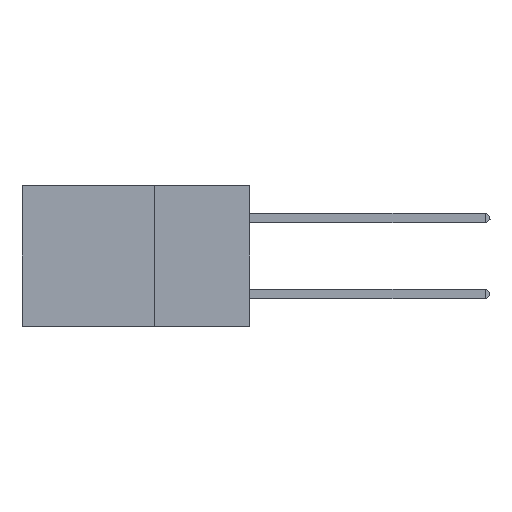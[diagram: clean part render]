
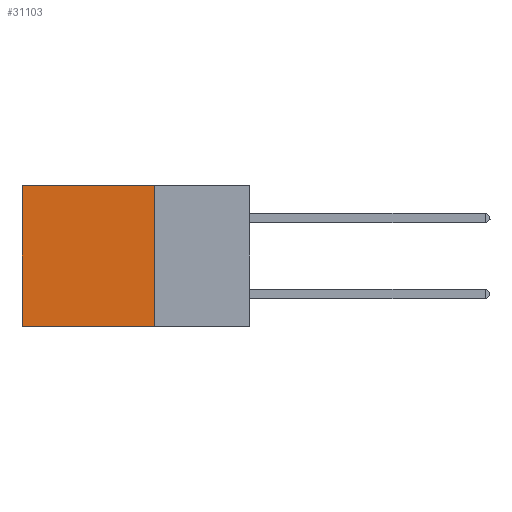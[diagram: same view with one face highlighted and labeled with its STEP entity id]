
A CAD part, left-side view. The second image highlights one B-rep face of the part: STEP entity #31103.
In plain terms, the highlighted planar face has unit normal (-1, 0, 0).
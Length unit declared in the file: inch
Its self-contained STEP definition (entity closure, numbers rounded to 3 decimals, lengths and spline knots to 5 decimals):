
#196 = DIRECTION ( 'NONE',  ( 0., 0., -1. ) ) ;
#592 = DIRECTION ( 'NONE',  ( 0., 0., -1. ) ) ;
#1498 = VERTEX_POINT ( 'NONE', #19120 ) ;
#3432 = EDGE_CURVE ( 'NONE', #1498, #26394, #28209, .T. ) ;
#7905 = AXIS2_PLACEMENT_3D ( 'NONE', #16651, #10890, #11061 ) ;
#9790 = VECTOR ( 'NONE', #32661, 39.37008 ) ;
#10890 = DIRECTION ( 'NONE',  ( 1., 0., 0. ) ) ;
#11061 = DIRECTION ( 'NONE',  ( 0., 0., -1. ) ) ;
#13774 = PLANE ( 'NONE',  #7905 ) ;
#13785 = LINE ( 'NONE', #26977, #15523 ) ;
#15254 = LINE ( 'NONE', #23399, #18573 ) ;
#15523 = VECTOR ( 'NONE', #592, 39.37008 ) ;
#16651 = CARTESIAN_POINT ( 'NONE',  ( 0.2875, 0.25, 0. ) ) ;
#17944 = EDGE_CURVE ( 'NONE', #27241, #30683, #20128, .T. ) ;
#18573 = VECTOR ( 'NONE', #196, 39.37008 ) ;
#19120 = CARTESIAN_POINT ( 'NONE',  ( 0.2875, 0.25, -0.37 ) ) ;
#19180 = FACE_OUTER_BOUND ( 'NONE', #29041, .T. ) ;
#20128 = LINE ( 'NONE', #30453, #9790 ) ;
#22042 = ORIENTED_EDGE ( 'NONE', *, *, #32487, .T. ) ;
#23048 = VECTOR ( 'NONE', #23655, 39.37008 ) ;
#23121 = EDGE_CURVE ( 'NONE', #27241, #1498, #15254, .T. ) ;
#23399 = CARTESIAN_POINT ( 'NONE',  ( 0.2875, 0.25, 0. ) ) ;
#23448 = CARTESIAN_POINT ( 'NONE',  ( 0.2875, 0.25, 0. ) ) ;
#23655 = DIRECTION ( 'NONE',  ( 0., 1., 0. ) ) ;
#23995 = CARTESIAN_POINT ( 'NONE',  ( 0.2875, 0.6, 0. ) ) ;
#26394 = VERTEX_POINT ( 'NONE', #29260 ) ;
#26977 = CARTESIAN_POINT ( 'NONE',  ( 0.2875, 0.6, 0. ) ) ;
#27241 = VERTEX_POINT ( 'NONE', #23448 ) ;
#28043 = CARTESIAN_POINT ( 'NONE',  ( 0.2875, 0.25, -0.37 ) ) ;
#28201 = ORIENTED_EDGE ( 'NONE', *, *, #17944, .T. ) ;
#28209 = LINE ( 'NONE', #28043, #23048 ) ;
#29041 = EDGE_LOOP ( 'NONE', ( #22042, #31644, #31750, #28201 ) ) ;
#29260 = CARTESIAN_POINT ( 'NONE',  ( 0.2875, 0.6, -0.37 ) ) ;
#30453 = CARTESIAN_POINT ( 'NONE',  ( 0.2875, 0.25, 0. ) ) ;
#30683 = VERTEX_POINT ( 'NONE', #23995 ) ;
#31103 = ADVANCED_FACE ( 'NONE', ( #19180 ), #13774, .F. ) ;
#31644 = ORIENTED_EDGE ( 'NONE', *, *, #3432, .F. ) ;
#31750 = ORIENTED_EDGE ( 'NONE', *, *, #23121, .F. ) ;
#32487 = EDGE_CURVE ( 'NONE', #30683, #26394, #13785, .T. ) ;
#32661 = DIRECTION ( 'NONE',  ( 0., 1., 0. ) ) ;
